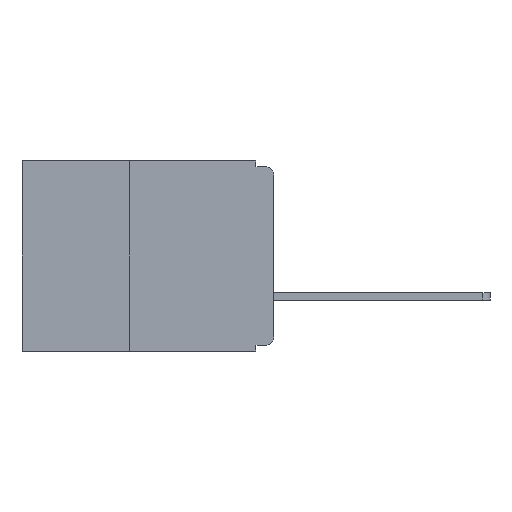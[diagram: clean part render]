
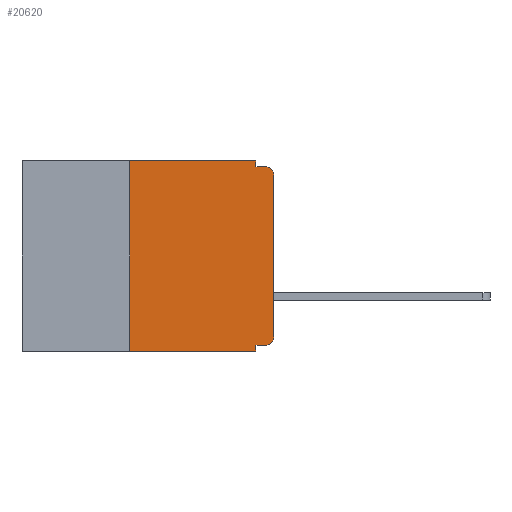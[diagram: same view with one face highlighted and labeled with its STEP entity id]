
A CAD part, left-side view. The second image highlights one B-rep face of the part: STEP entity #20620.
In plain terms, the highlighted planar face has unit normal (-1, 0, 0).
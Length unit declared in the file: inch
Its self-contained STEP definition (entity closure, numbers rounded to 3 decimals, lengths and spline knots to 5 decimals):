
#1077 = CARTESIAN_POINT ( 'NONE',  ( 0., 0., -0.01 ) ) ;
#1130 = ORIENTED_EDGE ( 'NONE', *, *, #3559, .T. ) ;
#1432 = ORIENTED_EDGE ( 'NONE', *, *, #25262, .T. ) ;
#1507 = AXIS2_PLACEMENT_3D ( 'NONE', #2336, #2254, #2231 ) ;
#1513 = VERTEX_POINT ( 'NONE', #2043 ) ;
#1971 = EDGE_CURVE ( 'NONE', #11625, #3693, #4108, .T. ) ;
#2043 = CARTESIAN_POINT ( 'NONE',  ( 0., 0.031, -0.01 ) ) ;
#2089 = CARTESIAN_POINT ( 'NONE',  ( 0., 0.437, 0. ) ) ;
#2231 = DIRECTION ( 'NONE',  ( 0., 0., -1. ) ) ;
#2254 = DIRECTION ( 'NONE',  ( -1., 0., 0. ) ) ;
#2336 = CARTESIAN_POINT ( 'NONE',  ( 0., 0.015, -0.305 ) ) ;
#2401 = DIRECTION ( 'NONE',  ( -1., 0., 0. ) ) ;
#2761 = ORIENTED_EDGE ( 'NONE', *, *, #1971, .F. ) ;
#3096 = VERTEX_POINT ( 'NONE', #12921 ) ;
#3460 = LINE ( 'NONE', #15904, #23841 ) ;
#3559 = EDGE_CURVE ( 'NONE', #19264, #7699, #7128, .T. ) ;
#3639 = ORIENTED_EDGE ( 'NONE', *, *, #13675, .T. ) ;
#3693 = VERTEX_POINT ( 'NONE', #8542 ) ;
#4108 = LINE ( 'NONE', #9863, #19300 ) ;
#4803 = EDGE_CURVE ( 'NONE', #16511, #21656, #20008, .T. ) ;
#5017 = AXIS2_PLACEMENT_3D ( 'NONE', #14334, #2401, #16292 ) ;
#5454 = LINE ( 'NONE', #1077, #14746 ) ;
#5739 = EDGE_CURVE ( 'NONE', #1513, #3096, #5454, .T. ) ;
#5998 = LINE ( 'NONE', #20301, #15892 ) ;
#6027 = FACE_OUTER_BOUND ( 'NONE', #12995, .T. ) ;
#6562 = CARTESIAN_POINT ( 'NONE',  ( 0., 0.25, -0.33 ) ) ;
#6627 = ORIENTED_EDGE ( 'NONE', *, *, #24556, .F. ) ;
#7060 = PLANE ( 'NONE',  #25209 ) ;
#7128 = CIRCLE ( 'NONE', #1507, 0.015 ) ;
#7699 = VERTEX_POINT ( 'NONE', #15714 ) ;
#8085 = ORIENTED_EDGE ( 'NONE', *, *, #17711, .F. ) ;
#8418 = CARTESIAN_POINT ( 'NONE',  ( 0., 0.015, -0.32 ) ) ;
#8542 = CARTESIAN_POINT ( 'NONE',  ( 0., 0.031, -0.33 ) ) ;
#9067 = DIRECTION ( 'NONE',  ( 0., 0., -1. ) ) ;
#9649 = DIRECTION ( 'NONE',  ( 0., 0., -1. ) ) ;
#9854 = CARTESIAN_POINT ( 'NONE',  ( 0., 0.031, 0. ) ) ;
#9863 = CARTESIAN_POINT ( 'NONE',  ( 0., 0.031, -0.33 ) ) ;
#9928 = DIRECTION ( 'NONE',  ( 0., 0., -1. ) ) ;
#10701 = LINE ( 'NONE', #21389, #21100 ) ;
#10782 = CARTESIAN_POINT ( 'NONE',  ( 0., 0.25, 0. ) ) ;
#11625 = VERTEX_POINT ( 'NONE', #23618 ) ;
#12089 = DIRECTION ( 'NONE',  ( 0., 1., 0. ) ) ;
#12133 = VERTEX_POINT ( 'NONE', #21397 ) ;
#12518 = DIRECTION ( 'NONE',  ( 0., 0., 1. ) ) ;
#12921 = CARTESIAN_POINT ( 'NONE',  ( 0., 0.015, -0.01 ) ) ;
#12995 = EDGE_LOOP ( 'NONE', ( #3639, #1432, #21898, #16790, #23894, #8085, #15309, #2761, #6627, #1130 ) ) ;
#13149 = CIRCLE ( 'NONE', #5017, 0.015 ) ;
#13395 = CARTESIAN_POINT ( 'NONE',  ( 0., 0., -0.025 ) ) ;
#13675 = EDGE_CURVE ( 'NONE', #7699, #17325, #5998, .T. ) ;
#14245 = DIRECTION ( 'NONE',  ( 0., -1., 0. ) ) ;
#14334 = CARTESIAN_POINT ( 'NONE',  ( 0., 0.015, -0.025 ) ) ;
#14746 = VECTOR ( 'NONE', #18964, 39.37008 ) ;
#14790 = VECTOR ( 'NONE', #15973, 39.37008 ) ;
#15309 = ORIENTED_EDGE ( 'NONE', *, *, #25236, .T. ) ;
#15476 = VECTOR ( 'NONE', #12518, 39.37008 ) ;
#15714 = CARTESIAN_POINT ( 'NONE',  ( 0., 0., -0.305 ) ) ;
#15892 = VECTOR ( 'NONE', #22266, 39.37008 ) ;
#15904 = CARTESIAN_POINT ( 'NONE',  ( 0., 0., -0.32 ) ) ;
#15973 = DIRECTION ( 'NONE',  ( 0., -1., 0. ) ) ;
#16134 = EDGE_CURVE ( 'NONE', #21656, #1513, #10701, .T. ) ;
#16209 = CARTESIAN_POINT ( 'NONE',  ( 0., 0.437, -0.33 ) ) ;
#16292 = DIRECTION ( 'NONE',  ( 0., 0., -1. ) ) ;
#16511 = VERTEX_POINT ( 'NONE', #10782 ) ;
#16790 = ORIENTED_EDGE ( 'NONE', *, *, #16134, .F. ) ;
#16895 = CARTESIAN_POINT ( 'NONE',  ( 0., 0.437, 0. ) ) ;
#17325 = VERTEX_POINT ( 'NONE', #13395 ) ;
#17711 = EDGE_CURVE ( 'NONE', #12133, #16511, #25250, .T. ) ;
#17716 = VECTOR ( 'NONE', #14245, 39.37008 ) ;
#18964 = DIRECTION ( 'NONE',  ( 0., -1., 0. ) ) ;
#19264 = VERTEX_POINT ( 'NONE', #8418 ) ;
#19300 = VECTOR ( 'NONE', #9928, 39.37008 ) ;
#20008 = LINE ( 'NONE', #2089, #14790 ) ;
#20301 = CARTESIAN_POINT ( 'NONE',  ( 0., 0., 0. ) ) ;
#20620 = ADVANCED_FACE ( 'NONE', ( #6027 ), #7060, .F. ) ;
#21100 = VECTOR ( 'NONE', #9649, 39.37008 ) ;
#21389 = CARTESIAN_POINT ( 'NONE',  ( 0., 0.031, 0. ) ) ;
#21397 = CARTESIAN_POINT ( 'NONE',  ( 0., 0.25, -0.33 ) ) ;
#21656 = VERTEX_POINT ( 'NONE', #9854 ) ;
#21898 = ORIENTED_EDGE ( 'NONE', *, *, #5739, .F. ) ;
#22266 = DIRECTION ( 'NONE',  ( 0., 0., 1. ) ) ;
#23519 = LINE ( 'NONE', #16209, #17716 ) ;
#23618 = CARTESIAN_POINT ( 'NONE',  ( 0., 0.031, -0.32 ) ) ;
#23841 = VECTOR ( 'NONE', #12089, 39.37008 ) ;
#23894 = ORIENTED_EDGE ( 'NONE', *, *, #4803, .F. ) ;
#24556 = EDGE_CURVE ( 'NONE', #19264, #11625, #3460, .T. ) ;
#24658 = DIRECTION ( 'NONE',  ( 1., 0., 0. ) ) ;
#25209 = AXIS2_PLACEMENT_3D ( 'NONE', #16895, #24658, #9067 ) ;
#25236 = EDGE_CURVE ( 'NONE', #12133, #3693, #23519, .T. ) ;
#25250 = LINE ( 'NONE', #6562, #15476 ) ;
#25262 = EDGE_CURVE ( 'NONE', #17325, #3096, #13149, .T. ) ;
